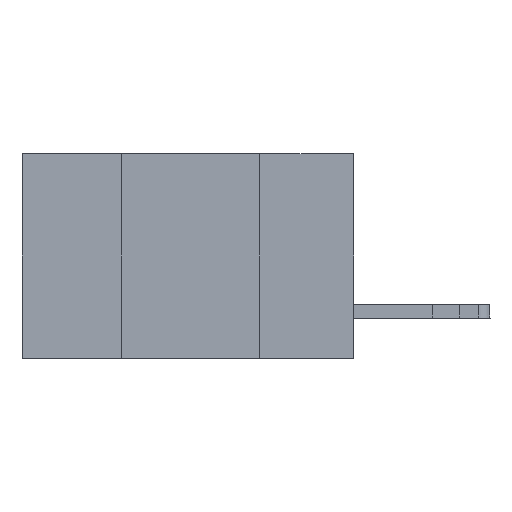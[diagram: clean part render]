
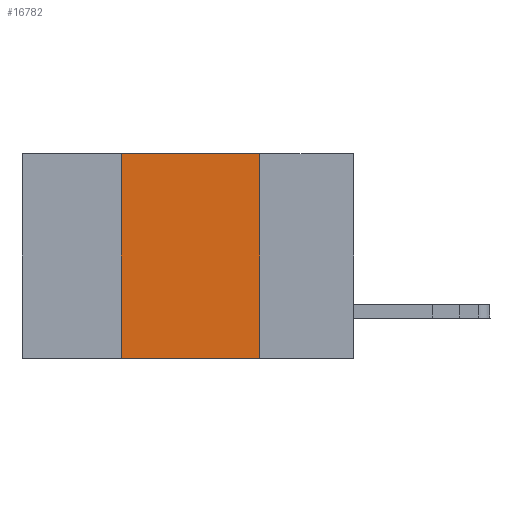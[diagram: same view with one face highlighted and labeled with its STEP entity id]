
A CAD part, left-side view. The second image highlights one B-rep face of the part: STEP entity #16782.
In plain terms, the highlighted planar face has unit normal (-1, 0, 0).
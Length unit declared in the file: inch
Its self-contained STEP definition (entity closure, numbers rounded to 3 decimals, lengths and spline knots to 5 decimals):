
#330 = DIRECTION ( 'NONE',  ( 0., 0., 1. ) ) ;
#375 = ORIENTED_EDGE ( 'NONE', *, *, #11222, .T. ) ;
#446 = CARTESIAN_POINT ( 'NONE',  ( 0., 0.42, 0. ) ) ;
#485 = LINE ( 'NONE', #24588, #29097 ) ;
#856 = VECTOR ( 'NONE', #330, 39.37008 ) ;
#1633 = CARTESIAN_POINT ( 'NONE',  ( 0., 0.17, 0. ) ) ;
#2314 = CARTESIAN_POINT ( 'NONE',  ( 0., 0.6, 0. ) ) ;
#2505 = DIRECTION ( 'NONE',  ( 0., 0., -1. ) ) ;
#3477 = CARTESIAN_POINT ( 'NONE',  ( 0., 0.6, -0.37 ) ) ;
#5605 = ORIENTED_EDGE ( 'NONE', *, *, #28595, .F. ) ;
#8981 = LINE ( 'NONE', #30022, #19853 ) ;
#9470 = DIRECTION ( 'NONE',  ( 0., -1., 0. ) ) ;
#10538 = ORIENTED_EDGE ( 'NONE', *, *, #37244, .F. ) ;
#11045 = PLANE ( 'NONE',  #11610 ) ;
#11222 = EDGE_CURVE ( 'NONE', #20387, #23184, #18443, .T. ) ;
#11610 = AXIS2_PLACEMENT_3D ( 'NONE', #2314, #29156, #2505 ) ;
#11983 = CARTESIAN_POINT ( 'NONE',  ( 0., 0.17, -0.37 ) ) ;
#14560 = VERTEX_POINT ( 'NONE', #1633 ) ;
#15218 = DIRECTION ( 'NONE',  ( 0., 0., -1. ) ) ;
#16782 = ADVANCED_FACE ( 'NONE', ( #25835 ), #11045, .F. ) ;
#18377 = EDGE_CURVE ( 'NONE', #37669, #14560, #485, .T. ) ;
#18443 = LINE ( 'NONE', #3477, #25842 ) ;
#19853 = VECTOR ( 'NONE', #15218, 39.37008 ) ;
#20387 = VERTEX_POINT ( 'NONE', #35040 ) ;
#21668 = DIRECTION ( 'NONE',  ( 0., -1., 0. ) ) ;
#23184 = VERTEX_POINT ( 'NONE', #11983 ) ;
#24433 = EDGE_LOOP ( 'NONE', ( #10538, #33360, #5605, #375 ) ) ;
#24588 = CARTESIAN_POINT ( 'NONE',  ( 0., 0.6, 0. ) ) ;
#25835 = FACE_OUTER_BOUND ( 'NONE', #24433, .T. ) ;
#25842 = VECTOR ( 'NONE', #9470, 39.37008 ) ;
#28595 = EDGE_CURVE ( 'NONE', #20387, #37669, #29318, .T. ) ;
#29097 = VECTOR ( 'NONE', #21668, 39.37008 ) ;
#29156 = DIRECTION ( 'NONE',  ( 1., 0., 0. ) ) ;
#29318 = LINE ( 'NONE', #35770, #856 ) ;
#30022 = CARTESIAN_POINT ( 'NONE',  ( 0., 0.17, 0. ) ) ;
#33360 = ORIENTED_EDGE ( 'NONE', *, *, #18377, .F. ) ;
#35040 = CARTESIAN_POINT ( 'NONE',  ( 0., 0.42, -0.37 ) ) ;
#35770 = CARTESIAN_POINT ( 'NONE',  ( 0., 0.42, 0. ) ) ;
#37244 = EDGE_CURVE ( 'NONE', #14560, #23184, #8981, .T. ) ;
#37669 = VERTEX_POINT ( 'NONE', #446 ) ;
